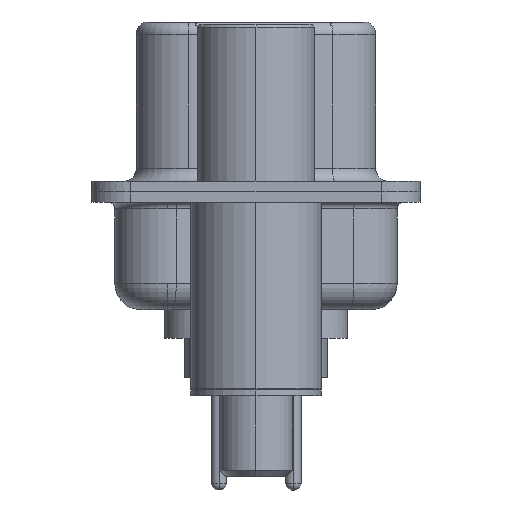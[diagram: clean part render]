
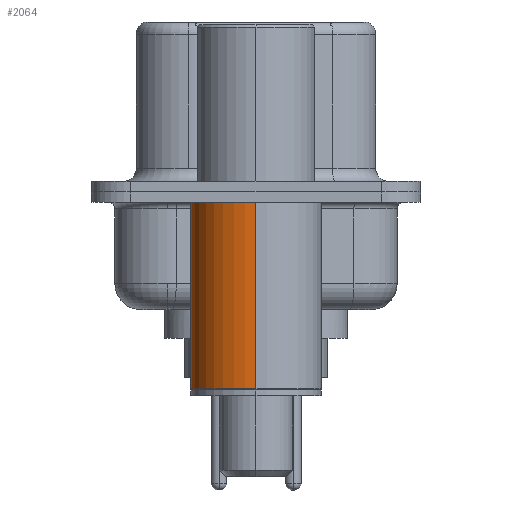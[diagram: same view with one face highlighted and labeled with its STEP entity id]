
A CAD part, left-side view. The second image highlights one B-rep face of the part: STEP entity #2064.
In plain terms, the highlighted cylindrical face has radius 2.5 mm (diameter 5 mm), a partial arc.
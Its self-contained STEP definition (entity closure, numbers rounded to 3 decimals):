
#548 = DIRECTION ( 'NONE',  ( 1., 0., 0. ) ) ;
#1214 = CIRCLE ( 'NONE', #10366, 2.5 ) ;
#1267 = EDGE_LOOP ( 'NONE', ( #8923, #17572, #8439, #14510 ) ) ;
#2064 = ADVANCED_FACE ( 'NONE', ( #25622 ), #24983, .T. ) ;
#2109 = CARTESIAN_POINT ( 'NONE',  ( 2.5, 0., -0.4 ) ) ;
#2707 = EDGE_CURVE ( 'NONE', #21131, #7781, #12368, .T. ) ;
#2900 = AXIS2_PLACEMENT_3D ( 'NONE', #18129, #6948, #6166 ) ;
#2965 = VECTOR ( 'NONE', #11183, 1000. ) ;
#4065 = CARTESIAN_POINT ( 'NONE',  ( -2.5, 0., -7.525 ) ) ;
#6166 = DIRECTION ( 'NONE',  ( 1., 0., 0. ) ) ;
#6396 = AXIS2_PLACEMENT_3D ( 'NONE', #24830, #12774, #548 ) ;
#6948 = DIRECTION ( 'NONE',  ( 0., 0., 1. ) ) ;
#7097 = VERTEX_POINT ( 'NONE', #4065 ) ;
#7781 = VERTEX_POINT ( 'NONE', #2109 ) ;
#8439 = ORIENTED_EDGE ( 'NONE', *, *, #17121, .F. ) ;
#8923 = ORIENTED_EDGE ( 'NONE', *, *, #23017, .T. ) ;
#9670 = CARTESIAN_POINT ( 'NONE',  ( -2.5, 0., -0.4 ) ) ;
#10066 = CARTESIAN_POINT ( 'NONE',  ( 0., 0., -7.525 ) ) ;
#10366 = AXIS2_PLACEMENT_3D ( 'NONE', #10066, #24161, #12121 ) ;
#11183 = DIRECTION ( 'NONE',  ( 0., 0., 1. ) ) ;
#11600 = CARTESIAN_POINT ( 'NONE',  ( 2.5, 0., 0.581 ) ) ;
#12121 = DIRECTION ( 'NONE',  ( 1., 0., 0. ) ) ;
#12368 = LINE ( 'NONE', #11600, #17085 ) ;
#12774 = DIRECTION ( 'NONE',  ( 0., 0., 1. ) ) ;
#14510 = ORIENTED_EDGE ( 'NONE', *, *, #2707, .F. ) ;
#14657 = CIRCLE ( 'NONE', #6396, 2.5 ) ;
#15794 = EDGE_CURVE ( 'NONE', #7097, #24220, #19095, .T. ) ;
#17085 = VECTOR ( 'NONE', #21513, 1000. ) ;
#17121 = EDGE_CURVE ( 'NONE', #7781, #24220, #14657, .T. ) ;
#17572 = ORIENTED_EDGE ( 'NONE', *, *, #15794, .T. ) ;
#17825 = CARTESIAN_POINT ( 'NONE',  ( 2.5, 0., -7.525 ) ) ;
#18129 = CARTESIAN_POINT ( 'NONE',  ( 0., 0., 0.581 ) ) ;
#19095 = LINE ( 'NONE', #21168, #2965 ) ;
#21131 = VERTEX_POINT ( 'NONE', #17825 ) ;
#21168 = CARTESIAN_POINT ( 'NONE',  ( -2.5, 0., 0.581 ) ) ;
#21513 = DIRECTION ( 'NONE',  ( 0., 0., 1. ) ) ;
#23017 = EDGE_CURVE ( 'NONE', #21131, #7097, #1214, .T. ) ;
#24161 = DIRECTION ( 'NONE',  ( 0., 0., 1. ) ) ;
#24220 = VERTEX_POINT ( 'NONE', #9670 ) ;
#24830 = CARTESIAN_POINT ( 'NONE',  ( 0., 0., -0.4 ) ) ;
#24983 = CYLINDRICAL_SURFACE ( 'NONE', #2900, 2.5 ) ;
#25622 = FACE_OUTER_BOUND ( 'NONE', #1267, .T. ) ;
